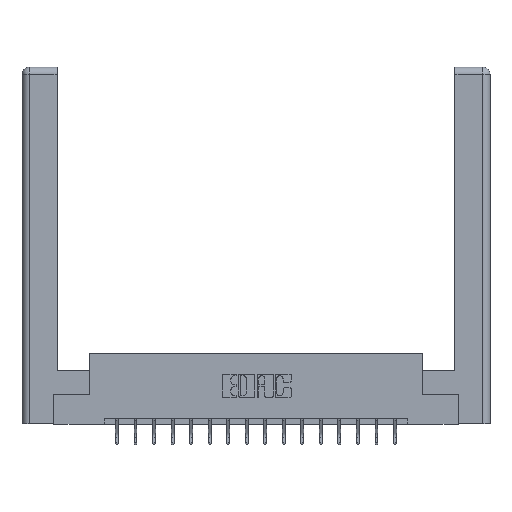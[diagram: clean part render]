
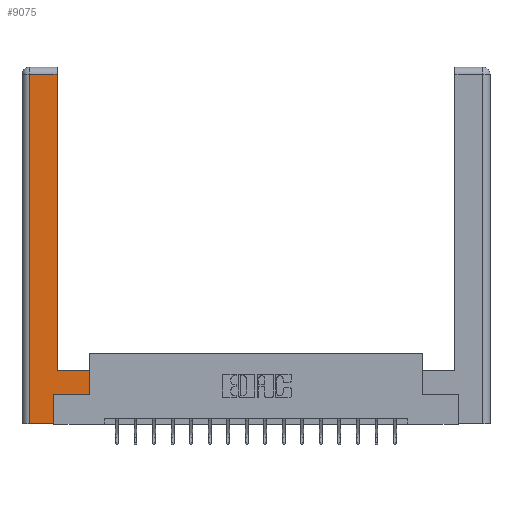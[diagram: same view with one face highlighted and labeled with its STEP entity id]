
A CAD part, top view. The second image highlights one B-rep face of the part: STEP entity #9075.
In plain terms, the highlighted planar face has unit normal (0, 0, 1).
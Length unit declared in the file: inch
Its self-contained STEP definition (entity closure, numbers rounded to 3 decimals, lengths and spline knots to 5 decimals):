
#13 = CARTESIAN_POINT ( 'NONE',  ( 0.0615, 2.94, 0. ) ) ;
#37 = VERTEX_POINT ( 'NONE', #902 ) ;
#251 = LINE ( 'NONE', #9191, #13965 ) ;
#836 = CARTESIAN_POINT ( 'NONE',  ( 0.295, 0.45, 0. ) ) ;
#902 = CARTESIAN_POINT ( 'NONE',  ( 0.565, 0.245, 0. ) ) ;
#916 = EDGE_CURVE ( 'NONE', #3748, #15215, #11088, .T. ) ;
#1103 = ORIENTED_EDGE ( 'NONE', *, *, #2169, .T. ) ;
#1451 = CARTESIAN_POINT ( 'NONE',  ( 0.0615, 0., 0. ) ) ;
#1713 = CARTESIAN_POINT ( 'NONE',  ( 0., 0., 0. ) ) ;
#1823 = VECTOR ( 'NONE', #9585, 39.37008 ) ;
#2114 = VECTOR ( 'NONE', #4364, 39.37008 ) ;
#2151 = CARTESIAN_POINT ( 'NONE',  ( 0.0615, 2.94, 0. ) ) ;
#2169 = EDGE_CURVE ( 'NONE', #3579, #37, #251, .T. ) ;
#2211 = CARTESIAN_POINT ( 'NONE',  ( 0.295, 2.94, 0. ) ) ;
#2212 = DIRECTION ( 'NONE',  ( -1., 0., 0. ) ) ;
#2276 = EDGE_CURVE ( 'NONE', #10967, #7072, #10581, .T. ) ;
#2334 = EDGE_CURVE ( 'NONE', #15215, #9162, #11468, .T. ) ;
#2371 = AXIS2_PLACEMENT_3D ( 'NONE', #1713, #13287, #3240 ) ;
#2486 = EDGE_CURVE ( 'NONE', #9162, #10967, #7713, .T. ) ;
#3135 = DIRECTION ( 'NONE',  ( 0., 1., 0. ) ) ;
#3240 = DIRECTION ( 'NONE',  ( -1., 0., 0. ) ) ;
#3579 = VERTEX_POINT ( 'NONE', #17497 ) ;
#3604 = ORIENTED_EDGE ( 'NONE', *, *, #9426, .T. ) ;
#3748 = VERTEX_POINT ( 'NONE', #8826 ) ;
#3881 = EDGE_LOOP ( 'NONE', ( #6739, #4251, #12903, #13030, #3604, #1103, #12348, #8020 ) ) ;
#4251 = ORIENTED_EDGE ( 'NONE', *, *, #2334, .T. ) ;
#4364 = DIRECTION ( 'NONE',  ( 0., -1., 0. ) ) ;
#4482 = LINE ( 'NONE', #6687, #10745 ) ;
#5402 = CARTESIAN_POINT ( 'NONE',  ( 0.295, 3., 0. ) ) ;
#6352 = CARTESIAN_POINT ( 'NONE',  ( 0.565, 0.45, 0. ) ) ;
#6545 = EDGE_CURVE ( 'NONE', #37, #8723, #8076, .T. ) ;
#6676 = EDGE_CURVE ( 'NONE', #8723, #3748, #17558, .T. ) ;
#6687 = CARTESIAN_POINT ( 'NONE',  ( 0.265, 0.245, 0. ) ) ;
#6739 = ORIENTED_EDGE ( 'NONE', *, *, #916, .T. ) ;
#7072 = VERTEX_POINT ( 'NONE', #10434 ) ;
#7400 = VECTOR ( 'NONE', #2212, 39.37008 ) ;
#7713 = LINE ( 'NONE', #1451, #2114 ) ;
#7866 = DIRECTION ( 'NONE',  ( 1., 0., 0. ) ) ;
#8020 = ORIENTED_EDGE ( 'NONE', *, *, #6676, .T. ) ;
#8076 = LINE ( 'NONE', #6352, #12801 ) ;
#8723 = VERTEX_POINT ( 'NONE', #12038 ) ;
#8826 = CARTESIAN_POINT ( 'NONE',  ( 0.295, 0.45, 0. ) ) ;
#9056 = PLANE ( 'NONE',  #2371 ) ;
#9075 = ADVANCED_FACE ( 'NONE', ( #16135 ), #9056, .F. ) ;
#9162 = VERTEX_POINT ( 'NONE', #13 ) ;
#9191 = CARTESIAN_POINT ( 'NONE',  ( 0.565, 0.245, 0. ) ) ;
#9426 = EDGE_CURVE ( 'NONE', #7072, #3579, #4482, .T. ) ;
#9585 = DIRECTION ( 'NONE',  ( -1., 0., 0. ) ) ;
#9937 = VECTOR ( 'NONE', #7866, 39.37008 ) ;
#10434 = CARTESIAN_POINT ( 'NONE',  ( 0.265, 0., 0. ) ) ;
#10581 = LINE ( 'NONE', #13797, #9937 ) ;
#10745 = VECTOR ( 'NONE', #3135, 39.37008 ) ;
#10967 = VERTEX_POINT ( 'NONE', #17646 ) ;
#11088 = LINE ( 'NONE', #5402, #17213 ) ;
#11227 = DIRECTION ( 'NONE',  ( 0., 1., 0. ) ) ;
#11468 = LINE ( 'NONE', #2151, #1823 ) ;
#12038 = CARTESIAN_POINT ( 'NONE',  ( 0.565, 0.45, 0. ) ) ;
#12348 = ORIENTED_EDGE ( 'NONE', *, *, #6545, .T. ) ;
#12801 = VECTOR ( 'NONE', #13413, 39.37008 ) ;
#12903 = ORIENTED_EDGE ( 'NONE', *, *, #2486, .T. ) ;
#13030 = ORIENTED_EDGE ( 'NONE', *, *, #2276, .T. ) ;
#13287 = DIRECTION ( 'NONE',  ( 0., 0., -1. ) ) ;
#13413 = DIRECTION ( 'NONE',  ( 0., 1., 0. ) ) ;
#13797 = CARTESIAN_POINT ( 'NONE',  ( 0.265, 0., 0. ) ) ;
#13965 = VECTOR ( 'NONE', #14945, 39.37008 ) ;
#14945 = DIRECTION ( 'NONE',  ( 1., 0., 0. ) ) ;
#15215 = VERTEX_POINT ( 'NONE', #2211 ) ;
#16135 = FACE_OUTER_BOUND ( 'NONE', #3881, .T. ) ;
#17213 = VECTOR ( 'NONE', #11227, 39.37008 ) ;
#17497 = CARTESIAN_POINT ( 'NONE',  ( 0.265, 0.245, 0. ) ) ;
#17558 = LINE ( 'NONE', #836, #7400 ) ;
#17646 = CARTESIAN_POINT ( 'NONE',  ( 0.0615, 0., 0. ) ) ;
